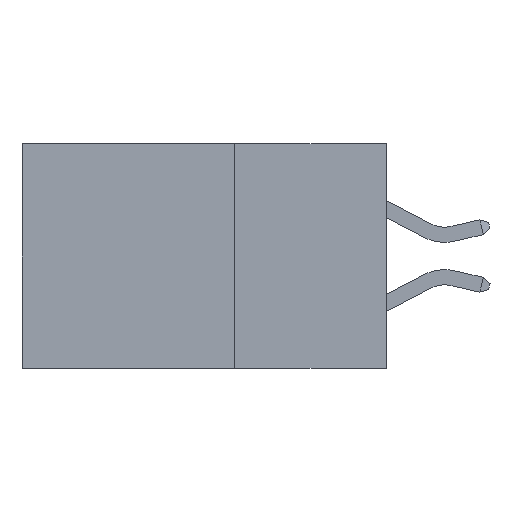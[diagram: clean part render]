
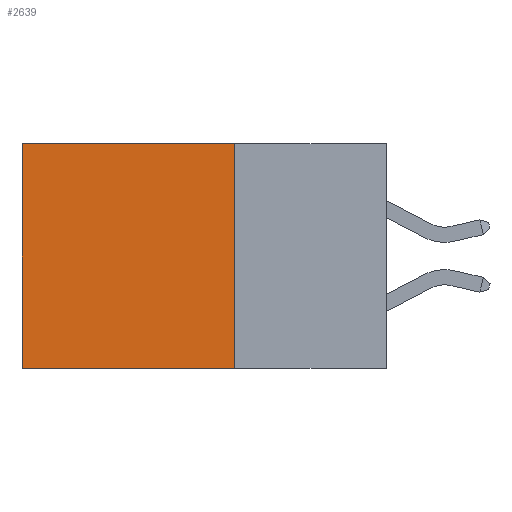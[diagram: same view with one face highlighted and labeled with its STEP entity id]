
A CAD part, left-side view. The second image highlights one B-rep face of the part: STEP entity #2639.
In plain terms, the highlighted planar face has unit normal (-1, 0, 0).
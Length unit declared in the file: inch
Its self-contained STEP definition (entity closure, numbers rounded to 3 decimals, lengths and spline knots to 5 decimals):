
#634 = LINE ( 'NONE', #5272, #5647 ) ;
#2313 = ORIENTED_EDGE ( 'NONE', *, *, #25093, .F. ) ;
#2639 = ADVANCED_FACE ( 'NONE', ( #3916 ), #11530, .F. ) ;
#2855 = VERTEX_POINT ( 'NONE', #15030 ) ;
#3467 = ORIENTED_EDGE ( 'NONE', *, *, #8397, .F. ) ;
#3566 = ORIENTED_EDGE ( 'NONE', *, *, #4331, .T. ) ;
#3916 = FACE_OUTER_BOUND ( 'NONE', #4026, .T. ) ;
#4026 = EDGE_LOOP ( 'NONE', ( #13695, #3467, #2313, #3566 ) ) ;
#4331 = EDGE_CURVE ( 'NONE', #26905, #24533, #24344, .T. ) ;
#5272 = CARTESIAN_POINT ( 'NONE',  ( 0.2615, 0.25, -0.37 ) ) ;
#5647 = VECTOR ( 'NONE', #9511, 39.37008 ) ;
#6267 = CARTESIAN_POINT ( 'NONE',  ( 0.2615, 0.25, -0.37 ) ) ;
#7829 = VECTOR ( 'NONE', #18601, 39.37008 ) ;
#8397 = EDGE_CURVE ( 'NONE', #2855, #20819, #23545, .T. ) ;
#9228 = AXIS2_PLACEMENT_3D ( 'NONE', #11304, #11252, #10910 ) ;
#9511 = DIRECTION ( 'NONE',  ( 0., 0., -1. ) ) ;
#10910 = DIRECTION ( 'NONE',  ( 0., 0., -1. ) ) ;
#11252 = DIRECTION ( 'NONE',  ( 1., 0., 0. ) ) ;
#11304 = CARTESIAN_POINT ( 'NONE',  ( 0.2615, 0.25, -0.37 ) ) ;
#11530 = PLANE ( 'NONE',  #9228 ) ;
#11827 = CARTESIAN_POINT ( 'NONE',  ( 0.2615, 0.6, 0. ) ) ;
#12678 = CARTESIAN_POINT ( 'NONE',  ( 0.2615, 0.6, -0.37 ) ) ;
#13215 = VECTOR ( 'NONE', #20851, 39.37008 ) ;
#13695 = ORIENTED_EDGE ( 'NONE', *, *, #24088, .T. ) ;
#14573 = VECTOR ( 'NONE', #20926, 39.37008 ) ;
#15030 = CARTESIAN_POINT ( 'NONE',  ( 0.2615, 0.25, -0.37 ) ) ;
#15867 = LINE ( 'NONE', #12678, #14573 ) ;
#16108 = CARTESIAN_POINT ( 'NONE',  ( 0.2615, 0.6, -0.37 ) ) ;
#18519 = CARTESIAN_POINT ( 'NONE',  ( 0.2615, 0.25, 0. ) ) ;
#18601 = DIRECTION ( 'NONE',  ( 0., 1., 0. ) ) ;
#19323 = CARTESIAN_POINT ( 'NONE',  ( 0.2615, 0.25, 0. ) ) ;
#20819 = VERTEX_POINT ( 'NONE', #16108 ) ;
#20851 = DIRECTION ( 'NONE',  ( 0., 1., 0. ) ) ;
#20926 = DIRECTION ( 'NONE',  ( 0., 0., -1. ) ) ;
#23545 = LINE ( 'NONE', #6267, #13215 ) ;
#24088 = EDGE_CURVE ( 'NONE', #24533, #20819, #15867, .T. ) ;
#24344 = LINE ( 'NONE', #18519, #7829 ) ;
#24533 = VERTEX_POINT ( 'NONE', #11827 ) ;
#25093 = EDGE_CURVE ( 'NONE', #26905, #2855, #634, .T. ) ;
#26905 = VERTEX_POINT ( 'NONE', #19323 ) ;
